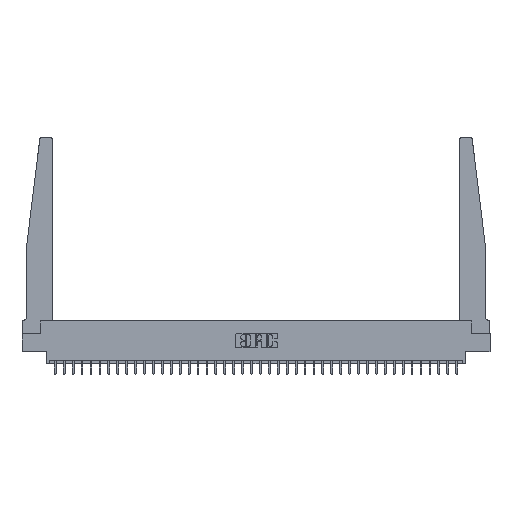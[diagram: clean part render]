
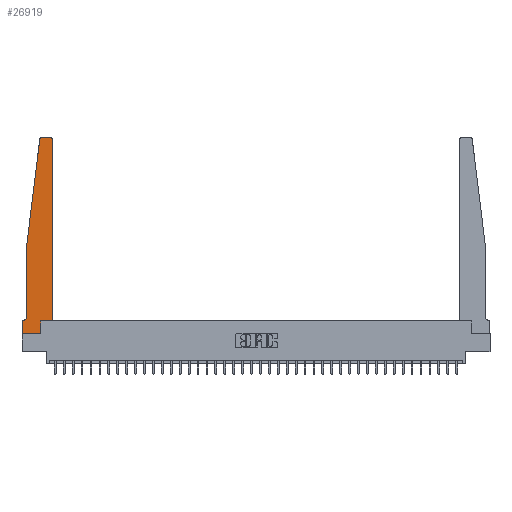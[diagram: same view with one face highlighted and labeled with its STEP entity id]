
A CAD part, top view. The second image highlights one B-rep face of the part: STEP entity #26919.
In plain terms, the highlighted planar face has unit normal (0, 0, 1).
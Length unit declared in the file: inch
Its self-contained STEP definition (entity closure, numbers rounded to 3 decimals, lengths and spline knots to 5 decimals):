
#21 = EDGE_LOOP ( 'NONE', ( #970, #7315, #1193, #857, #30228, #14656, #18427, #18477, #26407, #22956, #16005, #27035 ) ) ;
#508 = EDGE_CURVE ( 'NONE', #14820, #12046, #1890, .T. ) ;
#857 = ORIENTED_EDGE ( 'NONE', *, *, #17026, .T. ) ;
#970 = ORIENTED_EDGE ( 'NONE', *, *, #508, .T. ) ;
#1113 = VERTEX_POINT ( 'NONE', #12163 ) ;
#1193 = ORIENTED_EDGE ( 'NONE', *, *, #17756, .T. ) ;
#1210 = DIRECTION ( 'NONE',  ( 0., 0., 1. ) ) ;
#1890 = LINE ( 'NONE', #25309, #8241 ) ;
#2039 = VERTEX_POINT ( 'NONE', #24636 ) ;
#2047 = CARTESIAN_POINT ( 'NONE',  ( 0.2605, 0.18, 0.37 ) ) ;
#2227 = VECTOR ( 'NONE', #10999, 39.37008 ) ;
#2698 = CIRCLE ( 'NONE', #14669, 0.03 ) ;
#2876 = CARTESIAN_POINT ( 'NONE',  ( 0., 0., 0.37 ) ) ;
#3738 = CARTESIAN_POINT ( 'NONE',  ( 0.425, 0.18, 0.37 ) ) ;
#4051 = VECTOR ( 'NONE', #12870, 39.37008 ) ;
#4579 = VERTEX_POINT ( 'NONE', #28199 ) ;
#4600 = CARTESIAN_POINT ( 'NONE',  ( 0.425, 0.18, 0.37 ) ) ;
#5281 = CIRCLE ( 'NONE', #10191, 0.05 ) ;
#5851 = VERTEX_POINT ( 'NONE', #11916 ) ;
#6947 = CARTESIAN_POINT ( 'NONE',  ( 0.065, 1.25, 0.37 ) ) ;
#7066 = DIRECTION ( 'NONE',  ( 1., 0., 0. ) ) ;
#7315 = ORIENTED_EDGE ( 'NONE', *, *, #9224, .T. ) ;
#8112 = CARTESIAN_POINT ( 'NONE',  ( 0.27653, 2.72, 0.37 ) ) ;
#8241 = VECTOR ( 'NONE', #9421, 39.37008 ) ;
#8301 = DIRECTION ( 'NONE',  ( 0., -1., 0. ) ) ;
#8683 = CARTESIAN_POINT ( 'NONE',  ( 0.425, 0.18, 0.37 ) ) ;
#9224 = EDGE_CURVE ( 'NONE', #12046, #5851, #2698, .T. ) ;
#9421 = DIRECTION ( 'NONE',  ( -1., 0., 0. ) ) ;
#9860 = VECTOR ( 'NONE', #25993, 39.37008 ) ;
#9907 = EDGE_CURVE ( 'NONE', #4579, #2039, #31382, .T. ) ;
#10191 = AXIS2_PLACEMENT_3D ( 'NONE', #13565, #32053, #16250 ) ;
#10789 = DIRECTION ( 'NONE',  ( 1., 0., 0. ) ) ;
#10999 = DIRECTION ( 'NONE',  ( 1., 0., 0. ) ) ;
#11916 = CARTESIAN_POINT ( 'NONE',  ( 0.24675, 2.72367, 0.37 ) ) ;
#12046 = VERTEX_POINT ( 'NONE', #14849 ) ;
#12163 = CARTESIAN_POINT ( 'NONE',  ( 0.065, 0.2375, 0.37 ) ) ;
#12322 = PLANE ( 'NONE',  #13472 ) ;
#12420 = VERTEX_POINT ( 'NONE', #22990 ) ;
#12597 = CARTESIAN_POINT ( 'NONE',  ( 0.065, 1.25, 0.37 ) ) ;
#12667 = EDGE_CURVE ( 'NONE', #25826, #15487, #21316, .T. ) ;
#12870 = DIRECTION ( 'NONE',  ( 0., 1., 0. ) ) ;
#13169 = VERTEX_POINT ( 'NONE', #15172 ) ;
#13472 = AXIS2_PLACEMENT_3D ( 'NONE', #33472, #23020, #7066 ) ;
#13565 = CARTESIAN_POINT ( 'NONE',  ( 0.015, 0.2375, 0.37 ) ) ;
#13941 = LINE ( 'NONE', #18959, #19377 ) ;
#14271 = EDGE_CURVE ( 'NONE', #12420, #28152, #30717, .T. ) ;
#14656 = ORIENTED_EDGE ( 'NONE', *, *, #12667, .T. ) ;
#14669 = AXIS2_PLACEMENT_3D ( 'NONE', #8112, #26661, #10789 ) ;
#14820 = VERTEX_POINT ( 'NONE', #29867 ) ;
#14849 = CARTESIAN_POINT ( 'NONE',  ( 0.27653, 2.75, 0.37 ) ) ;
#15172 = CARTESIAN_POINT ( 'NONE',  ( 0.425, 2.72, 0.37 ) ) ;
#15487 = VERTEX_POINT ( 'NONE', #16802 ) ;
#16005 = ORIENTED_EDGE ( 'NONE', *, *, #27366, .T. ) ;
#16250 = DIRECTION ( 'NONE',  ( -1., 0., 0. ) ) ;
#16528 = EDGE_CURVE ( 'NONE', #2039, #12420, #33139, .T. ) ;
#16802 = CARTESIAN_POINT ( 'NONE',  ( 0., 0.1875, 0.37 ) ) ;
#17026 = EDGE_CURVE ( 'NONE', #30499, #1113, #31479, .T. ) ;
#17222 = DIRECTION ( 'NONE',  ( 1., 0., 0. ) ) ;
#17325 = CARTESIAN_POINT ( 'NONE',  ( 0.395, 2.72, 0.37 ) ) ;
#17756 = EDGE_CURVE ( 'NONE', #5851, #30499, #23989, .T. ) ;
#18225 = CIRCLE ( 'NONE', #28753, 0.03 ) ;
#18427 = ORIENTED_EDGE ( 'NONE', *, *, #19547, .T. ) ;
#18477 = ORIENTED_EDGE ( 'NONE', *, *, #9907, .T. ) ;
#18959 = CARTESIAN_POINT ( 'NONE',  ( 0., 0., 0.37 ) ) ;
#19377 = VECTOR ( 'NONE', #8301, 39.37008 ) ;
#19547 = EDGE_CURVE ( 'NONE', #15487, #4579, #13941, .T. ) ;
#20010 = DIRECTION ( 'NONE',  ( 1., 0., 0. ) ) ;
#20665 = DIRECTION ( 'NONE',  ( 0., -1., 0. ) ) ;
#21316 = LINE ( 'NONE', #31855, #27791 ) ;
#21531 = VECTOR ( 'NONE', #24591, 39.37008 ) ;
#22956 = ORIENTED_EDGE ( 'NONE', *, *, #14271, .T. ) ;
#22990 = CARTESIAN_POINT ( 'NONE',  ( 0.2605, 0.18, 0.37 ) ) ;
#23020 = DIRECTION ( 'NONE',  ( 0., 0., 1. ) ) ;
#23357 = CARTESIAN_POINT ( 'NONE',  ( 0.065, 1.25, 0.37 ) ) ;
#23635 = VECTOR ( 'NONE', #20665, 39.37008 ) ;
#23989 = LINE ( 'NONE', #23357, #9860 ) ;
#24591 = DIRECTION ( 'NONE',  ( 0., 1., 0. ) ) ;
#24636 = CARTESIAN_POINT ( 'NONE',  ( 0.2605, 0., 0.37 ) ) ;
#25309 = CARTESIAN_POINT ( 'NONE',  ( 0.25, 2.75, 0.37 ) ) ;
#25771 = DIRECTION ( 'NONE',  ( -1., 0., 0. ) ) ;
#25826 = VERTEX_POINT ( 'NONE', #31948 ) ;
#25993 = DIRECTION ( 'NONE',  ( -0.122, -0.992, 0. ) ) ;
#26407 = ORIENTED_EDGE ( 'NONE', *, *, #16528, .T. ) ;
#26661 = DIRECTION ( 'NONE',  ( 0., 0., 1. ) ) ;
#26919 = ADVANCED_FACE ( 'NONE', ( #29363 ), #12322, .T. ) ;
#27035 = ORIENTED_EDGE ( 'NONE', *, *, #27528, .T. ) ;
#27366 = EDGE_CURVE ( 'NONE', #28152, #13169, #28502, .T. ) ;
#27528 = EDGE_CURVE ( 'NONE', #13169, #14820, #18225, .T. ) ;
#27791 = VECTOR ( 'NONE', #25771, 39.37008 ) ;
#28152 = VERTEX_POINT ( 'NONE', #4600 ) ;
#28199 = CARTESIAN_POINT ( 'NONE',  ( 0., 0., 0.37 ) ) ;
#28502 = LINE ( 'NONE', #8683, #21531 ) ;
#28753 = AXIS2_PLACEMENT_3D ( 'NONE', #17325, #1210, #20010 ) ;
#29049 = VECTOR ( 'NONE', #17222, 39.37008 ) ;
#29363 = FACE_OUTER_BOUND ( 'NONE', #21, .T. ) ;
#29867 = CARTESIAN_POINT ( 'NONE',  ( 0.395, 2.75, 0.37 ) ) ;
#30228 = ORIENTED_EDGE ( 'NONE', *, *, #31429, .T. ) ;
#30499 = VERTEX_POINT ( 'NONE', #6947 ) ;
#30717 = LINE ( 'NONE', #3738, #29049 ) ;
#31382 = LINE ( 'NONE', #2876, #2227 ) ;
#31429 = EDGE_CURVE ( 'NONE', #1113, #25826, #5281, .T. ) ;
#31479 = LINE ( 'NONE', #12597, #23635 ) ;
#31855 = CARTESIAN_POINT ( 'NONE',  ( 0.065, 0.1875, 0.37 ) ) ;
#31948 = CARTESIAN_POINT ( 'NONE',  ( 0.015, 0.1875, 0.37 ) ) ;
#32053 = DIRECTION ( 'NONE',  ( 0., 0., -1. ) ) ;
#33139 = LINE ( 'NONE', #2047, #4051 ) ;
#33472 = CARTESIAN_POINT ( 'NONE',  ( 0., 0.1875, 0.37 ) ) ;
